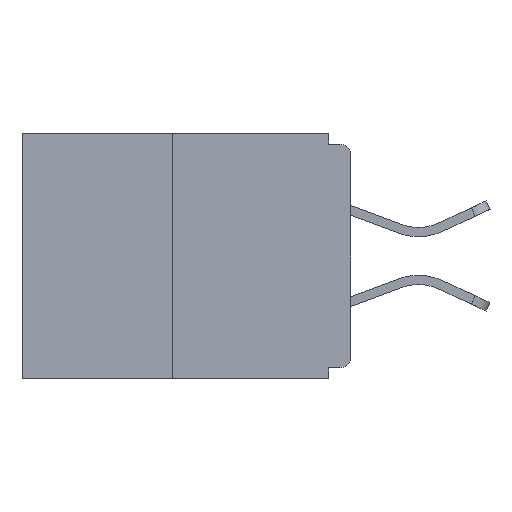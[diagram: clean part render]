
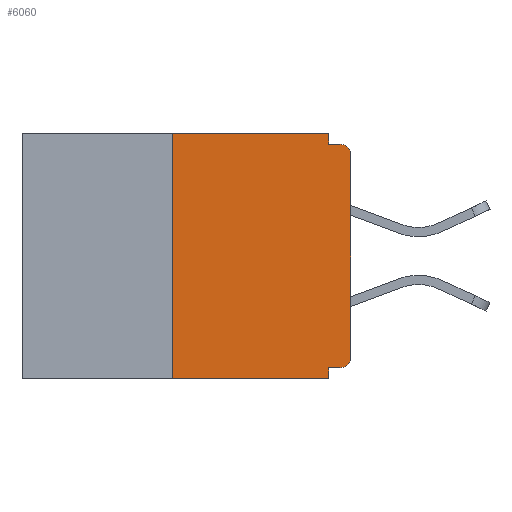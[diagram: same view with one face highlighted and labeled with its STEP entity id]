
A CAD part, left-side view. The second image highlights one B-rep face of the part: STEP entity #6060.
In plain terms, the highlighted planar face has unit normal (-1, 0, 0).
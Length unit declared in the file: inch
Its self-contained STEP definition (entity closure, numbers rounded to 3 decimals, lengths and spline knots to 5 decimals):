
#95 = DIRECTION ( 'NONE',  ( 0., 1., 0. ) ) ;
#136 = DIRECTION ( 'NONE',  ( -1., 0., 0. ) ) ;
#349 = CARTESIAN_POINT ( 'NONE',  ( 0., 0.015, -0.328 ) ) ;
#398 = CARTESIAN_POINT ( 'NONE',  ( 0., 0.25, 0. ) ) ;
#525 = VERTEX_POINT ( 'NONE', #5498 ) ;
#644 = LINE ( 'NONE', #398, #7697 ) ;
#667 = LINE ( 'NONE', #7655, #8745 ) ;
#761 = EDGE_CURVE ( 'NONE', #2431, #1872, #1234, .T. ) ;
#907 = EDGE_CURVE ( 'NONE', #525, #9672, #667, .T. ) ;
#971 = CARTESIAN_POINT ( 'NONE',  ( 0., 0.031, -0.328 ) ) ;
#1234 = LINE ( 'NONE', #9999, #9984 ) ;
#1473 = CARTESIAN_POINT ( 'NONE',  ( 0., 0.46, 0. ) ) ;
#1538 = DIRECTION ( 'NONE',  ( 0., 0., -1. ) ) ;
#1701 = VECTOR ( 'NONE', #95, 39.37008 ) ;
#1778 = VERTEX_POINT ( 'NONE', #6921 ) ;
#1872 = VERTEX_POINT ( 'NONE', #11177 ) ;
#2086 = VECTOR ( 'NONE', #9844, 39.37008 ) ;
#2420 = CARTESIAN_POINT ( 'NONE',  ( 0., 0.031, 0. ) ) ;
#2431 = VERTEX_POINT ( 'NONE', #6952 ) ;
#2470 = FACE_OUTER_BOUND ( 'NONE', #10202, .T. ) ;
#2538 = DIRECTION ( 'NONE',  ( 0., 0., -1. ) ) ;
#2566 = LINE ( 'NONE', #6121, #8605 ) ;
#2633 = ORIENTED_EDGE ( 'NONE', *, *, #907, .F. ) ;
#2745 = CIRCLE ( 'NONE', #7594, 0.015 ) ;
#3009 = LINE ( 'NONE', #9438, #10419 ) ;
#3029 = VECTOR ( 'NONE', #2538, 39.37008 ) ;
#3084 = EDGE_CURVE ( 'NONE', #7360, #6809, #6283, .T. ) ;
#3939 = VERTEX_POINT ( 'NONE', #349 ) ;
#4010 = ORIENTED_EDGE ( 'NONE', *, *, #5526, .F. ) ;
#4087 = DIRECTION ( 'NONE',  ( 0., -1., 0. ) ) ;
#4108 = EDGE_CURVE ( 'NONE', #8226, #1778, #2566, .T. ) ;
#4412 = EDGE_CURVE ( 'NONE', #3939, #7113, #6213, .T. ) ;
#4495 = DIRECTION ( 'NONE',  ( 0., 0., -1. ) ) ;
#4667 = DIRECTION ( 'NONE',  ( 0., 0., -1. ) ) ;
#4920 = PLANE ( 'NONE',  #9695 ) ;
#5065 = CARTESIAN_POINT ( 'NONE',  ( 0., 0., -0.328 ) ) ;
#5498 = CARTESIAN_POINT ( 'NONE',  ( 0., 0.25, 0. ) ) ;
#5526 = EDGE_CURVE ( 'NONE', #7113, #1872, #3009, .T. ) ;
#5529 = ORIENTED_EDGE ( 'NONE', *, *, #3084, .T. ) ;
#5541 = ORIENTED_EDGE ( 'NONE', *, *, #4412, .F. ) ;
#5631 = CARTESIAN_POINT ( 'NONE',  ( 0., 0., -0.03 ) ) ;
#6034 = CARTESIAN_POINT ( 'NONE',  ( 0., 0., -0.313 ) ) ;
#6060 = ADVANCED_FACE ( 'NONE', ( #2470 ), #4920, .F. ) ;
#6121 = CARTESIAN_POINT ( 'NONE',  ( 0., 0., -0.015 ) ) ;
#6154 = LINE ( 'NONE', #10538, #3029 ) ;
#6199 = CARTESIAN_POINT ( 'NONE',  ( 0., 0.015, -0.03 ) ) ;
#6213 = LINE ( 'NONE', #5065, #1701 ) ;
#6283 = LINE ( 'NONE', #10892, #2086 ) ;
#6353 = AXIS2_PLACEMENT_3D ( 'NONE', #9112, #136, #4667 ) ;
#6397 = EDGE_CURVE ( 'NONE', #3939, #7360, #10276, .T. ) ;
#6757 = DIRECTION ( 'NONE',  ( 0., 0., -1. ) ) ;
#6809 = VERTEX_POINT ( 'NONE', #5631 ) ;
#6921 = CARTESIAN_POINT ( 'NONE',  ( 0., 0.015, -0.015 ) ) ;
#6952 = CARTESIAN_POINT ( 'NONE',  ( 0., 0.25, -0.343 ) ) ;
#7113 = VERTEX_POINT ( 'NONE', #971 ) ;
#7205 = ORIENTED_EDGE ( 'NONE', *, *, #4108, .F. ) ;
#7311 = DIRECTION ( 'NONE',  ( 0., -1., 0. ) ) ;
#7360 = VERTEX_POINT ( 'NONE', #6034 ) ;
#7512 = DIRECTION ( 'NONE',  ( 0., 0., 1. ) ) ;
#7594 = AXIS2_PLACEMENT_3D ( 'NONE', #6199, #9649, #4495 ) ;
#7635 = ORIENTED_EDGE ( 'NONE', *, *, #9101, .F. ) ;
#7655 = CARTESIAN_POINT ( 'NONE',  ( 0., 0.46, 0. ) ) ;
#7697 = VECTOR ( 'NONE', #7512, 39.37008 ) ;
#8226 = VERTEX_POINT ( 'NONE', #9421 ) ;
#8605 = VECTOR ( 'NONE', #9693, 39.37008 ) ;
#8610 = ORIENTED_EDGE ( 'NONE', *, *, #761, .T. ) ;
#8667 = DIRECTION ( 'NONE',  ( 1., 0., 0. ) ) ;
#8745 = VECTOR ( 'NONE', #4087, 39.37008 ) ;
#9101 = EDGE_CURVE ( 'NONE', #2431, #525, #644, .T. ) ;
#9112 = CARTESIAN_POINT ( 'NONE',  ( 0., 0.015, -0.313 ) ) ;
#9169 = ORIENTED_EDGE ( 'NONE', *, *, #6397, .T. ) ;
#9343 = ORIENTED_EDGE ( 'NONE', *, *, #11195, .T. ) ;
#9421 = CARTESIAN_POINT ( 'NONE',  ( 0., 0.031, -0.015 ) ) ;
#9438 = CARTESIAN_POINT ( 'NONE',  ( 0., 0.031, -0.343 ) ) ;
#9589 = ORIENTED_EDGE ( 'NONE', *, *, #9660, .F. ) ;
#9649 = DIRECTION ( 'NONE',  ( -1., 0., 0. ) ) ;
#9660 = EDGE_CURVE ( 'NONE', #9672, #8226, #6154, .T. ) ;
#9672 = VERTEX_POINT ( 'NONE', #2420 ) ;
#9693 = DIRECTION ( 'NONE',  ( 0., -1., 0. ) ) ;
#9695 = AXIS2_PLACEMENT_3D ( 'NONE', #1473, #8667, #1538 ) ;
#9844 = DIRECTION ( 'NONE',  ( 0., 0., 1. ) ) ;
#9984 = VECTOR ( 'NONE', #7311, 39.37008 ) ;
#9999 = CARTESIAN_POINT ( 'NONE',  ( 0., 0.46, -0.343 ) ) ;
#10202 = EDGE_LOOP ( 'NONE', ( #2633, #7635, #8610, #4010, #5541, #9169, #5529, #9343, #7205, #9589 ) ) ;
#10276 = CIRCLE ( 'NONE', #6353, 0.015 ) ;
#10419 = VECTOR ( 'NONE', #6757, 39.37008 ) ;
#10538 = CARTESIAN_POINT ( 'NONE',  ( 0., 0.031, 0. ) ) ;
#10892 = CARTESIAN_POINT ( 'NONE',  ( 0., 0., 0. ) ) ;
#11177 = CARTESIAN_POINT ( 'NONE',  ( 0., 0.031, -0.343 ) ) ;
#11195 = EDGE_CURVE ( 'NONE', #6809, #1778, #2745, .T. ) ;
